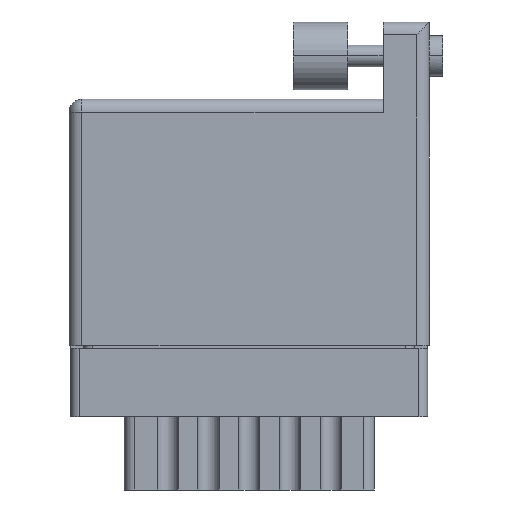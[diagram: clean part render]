
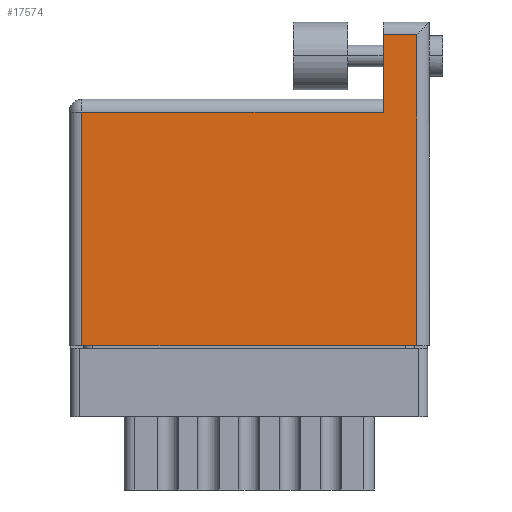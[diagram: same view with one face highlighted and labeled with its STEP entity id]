
A CAD part, front view. The second image highlights one B-rep face of the part: STEP entity #17574.
In plain terms, the highlighted face is planar.
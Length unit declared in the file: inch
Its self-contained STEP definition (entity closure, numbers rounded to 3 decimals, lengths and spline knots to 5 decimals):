
#913 = CARTESIAN_POINT ( 'NONE',  ( 1.155, 1.143, 0. ) ) ;
#1563 = DIRECTION ( 'NONE',  ( 1., 0., 0. ) ) ;
#1779 = CARTESIAN_POINT ( 'NONE',  ( 0., 0., 0. ) ) ;
#2006 = LINE ( 'NONE', #24769, #23668 ) ;
#2052 = ORIENTED_EDGE ( 'NONE', *, *, #27284, .T. ) ;
#3451 = VERTEX_POINT ( 'NONE', #913 ) ;
#4019 = VECTOR ( 'NONE', #18608, 39.37008 ) ;
#4398 = EDGE_CURVE ( 'NONE', #4764, #3451, #22766, .T. ) ;
#4450 = DIRECTION ( 'NONE',  ( 0., -1., 0. ) ) ;
#4758 = CARTESIAN_POINT ( 'NONE',  ( 0.047, 0., 0. ) ) ;
#4764 = VERTEX_POINT ( 'NONE', #20529 ) ;
#5018 = VECTOR ( 'NONE', #5581, 39.37008 ) ;
#5273 = VERTEX_POINT ( 'NONE', #25492 ) ;
#5581 = DIRECTION ( 'NONE',  ( -1., 0., 0. ) ) ;
#6231 = VERTEX_POINT ( 'NONE', #26187 ) ;
#10747 = EDGE_CURVE ( 'NONE', #3451, #5273, #17182, .T. ) ;
#11923 = EDGE_CURVE ( 'NONE', #5273, #17359, #19364, .T. ) ;
#12183 = ORIENTED_EDGE ( 'NONE', *, *, #4398, .T. ) ;
#13270 = EDGE_LOOP ( 'NONE', ( #13759, #2052, #12183, #23420, #20581, #23276 ) ) ;
#13603 = EDGE_CURVE ( 'NONE', #17359, #6231, #21477, .T. ) ;
#13759 = ORIENTED_EDGE ( 'NONE', *, *, #27419, .T. ) ;
#13858 = CARTESIAN_POINT ( 'NONE',  ( 1.155, 1.143, 0. ) ) ;
#14188 = DIRECTION ( 'NONE',  ( 0., -1., 0. ) ) ;
#14398 = CARTESIAN_POINT ( 'NONE',  ( 1.278, 0., 0. ) ) ;
#15012 = CARTESIAN_POINT ( 'NONE',  ( 0., 0.906, 0. ) ) ;
#16106 = FACE_OUTER_BOUND ( 'NONE', #13270, .T. ) ;
#17182 = LINE ( 'NONE', #20908, #19413 ) ;
#17359 = VERTEX_POINT ( 'NONE', #21130 ) ;
#17574 = ADVANCED_FACE ( 'NONE', ( #16106 ), #26499, .F. ) ;
#17602 = DIRECTION ( 'NONE',  ( 0., 0., -1. ) ) ;
#17676 = CARTESIAN_POINT ( 'NONE',  ( 0., 0.859, 0. ) ) ;
#17787 = VECTOR ( 'NONE', #4450, 39.37008 ) ;
#18608 = DIRECTION ( 'NONE',  ( -1., 0., 0. ) ) ;
#19364 = LINE ( 'NONE', #17676, #5018 ) ;
#19413 = VECTOR ( 'NONE', #14188, 39.37008 ) ;
#20159 = DIRECTION ( 'NONE',  ( 0., 1., 0. ) ) ;
#20529 = CARTESIAN_POINT ( 'NONE',  ( 1.278, 1.143, 0. ) ) ;
#20581 = ORIENTED_EDGE ( 'NONE', *, *, #11923, .T. ) ;
#20908 = CARTESIAN_POINT ( 'NONE',  ( 1.155, 1.19, 0. ) ) ;
#21130 = CARTESIAN_POINT ( 'NONE',  ( 0.047, 0.859, 0. ) ) ;
#21477 = LINE ( 'NONE', #4758, #17787 ) ;
#21827 = AXIS2_PLACEMENT_3D ( 'NONE', #15012, #17602, #21918 ) ;
#21918 = DIRECTION ( 'NONE',  ( -1., 0., 0. ) ) ;
#22766 = LINE ( 'NONE', #13858, #4019 ) ;
#23276 = ORIENTED_EDGE ( 'NONE', *, *, #13603, .T. ) ;
#23420 = ORIENTED_EDGE ( 'NONE', *, *, #10747, .T. ) ;
#23668 = VECTOR ( 'NONE', #20159, 39.37008 ) ;
#24769 = CARTESIAN_POINT ( 'NONE',  ( 1.278, 1.19, 0. ) ) ;
#24770 = VECTOR ( 'NONE', #1563, 39.37008 ) ;
#25492 = CARTESIAN_POINT ( 'NONE',  ( 1.155, 0.859, 0. ) ) ;
#26187 = CARTESIAN_POINT ( 'NONE',  ( 0.047, 0., 0. ) ) ;
#26220 = LINE ( 'NONE', #1779, #24770 ) ;
#26499 = PLANE ( 'NONE',  #21827 ) ;
#27284 = EDGE_CURVE ( 'NONE', #28888, #4764, #2006, .T. ) ;
#27419 = EDGE_CURVE ( 'NONE', #6231, #28888, #26220, .T. ) ;
#28888 = VERTEX_POINT ( 'NONE', #14398 ) ;
